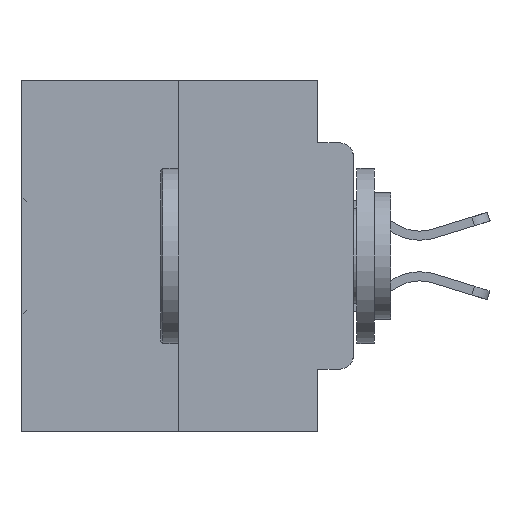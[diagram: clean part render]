
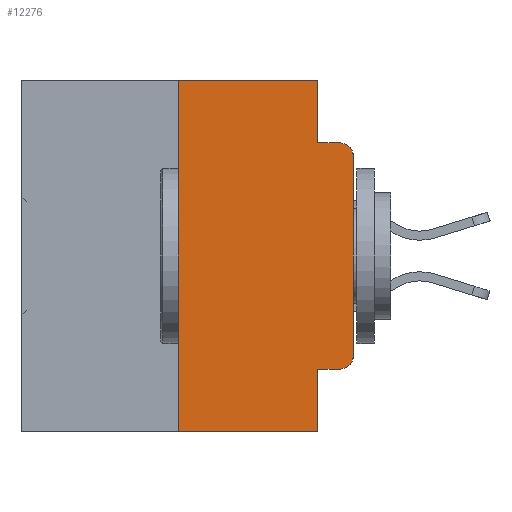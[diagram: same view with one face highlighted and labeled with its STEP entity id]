
A CAD part, left-side view. The second image highlights one B-rep face of the part: STEP entity #12276.
In plain terms, the highlighted planar face has unit normal (-1, 0, 0).
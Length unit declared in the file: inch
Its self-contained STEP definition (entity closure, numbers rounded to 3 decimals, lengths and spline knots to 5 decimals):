
#184 = CARTESIAN_POINT ( 'NONE',  ( 0., 0.02, -0.4115 ) ) ;
#1224 = AXIS2_PLACEMENT_3D ( 'NONE', #18841, #11108, #29218 ) ;
#1519 = ORIENTED_EDGE ( 'NONE', *, *, #25616, .T. ) ;
#1981 = ORIENTED_EDGE ( 'NONE', *, *, #29517, .F. ) ;
#2162 = DIRECTION ( 'NONE',  ( 0., -1., 0. ) ) ;
#2672 = CIRCLE ( 'NONE', #17789, 0.02 ) ;
#2979 = CARTESIAN_POINT ( 'NONE',  ( 0., 0.051, -0.0885 ) ) ;
#3383 = LINE ( 'NONE', #22987, #22512 ) ;
#3683 = VECTOR ( 'NONE', #31004, 39.37008 ) ;
#4195 = CARTESIAN_POINT ( 'NONE',  ( 0., 0., -0.1085 ) ) ;
#4209 = LINE ( 'NONE', #6127, #18863 ) ;
#4458 = CARTESIAN_POINT ( 'NONE',  ( 0., 0.02, -0.1085 ) ) ;
#4863 = VERTEX_POINT ( 'NONE', #7404 ) ;
#4993 = LINE ( 'NONE', #8942, #24950 ) ;
#5609 = DIRECTION ( 'NONE',  ( 0., -1., 0. ) ) ;
#5729 = VECTOR ( 'NONE', #16013, 39.37008 ) ;
#5787 = VERTEX_POINT ( 'NONE', #30250 ) ;
#5903 = VERTEX_POINT ( 'NONE', #7399 ) ;
#6127 = CARTESIAN_POINT ( 'NONE',  ( 0., 0.051, 0. ) ) ;
#6331 = CARTESIAN_POINT ( 'NONE',  ( 0., 0.02, -0.0885 ) ) ;
#6357 = DIRECTION ( 'NONE',  ( 0., 0., 1. ) ) ;
#6888 = LINE ( 'NONE', #2979, #33514 ) ;
#7072 = DIRECTION ( 'NONE',  ( 0., 0., -1. ) ) ;
#7381 = EDGE_CURVE ( 'NONE', #21571, #5903, #15150, .T. ) ;
#7399 = CARTESIAN_POINT ( 'NONE',  ( 0., 0.051, -0.5 ) ) ;
#7404 = CARTESIAN_POINT ( 'NONE',  ( 0., 0.051, -0.0885 ) ) ;
#7880 = FACE_OUTER_BOUND ( 'NONE', #33352, .T. ) ;
#8194 = VECTOR ( 'NONE', #9558, 39.37008 ) ;
#8215 = EDGE_CURVE ( 'NONE', #5787, #15349, #24443, .T. ) ;
#8376 = PLANE ( 'NONE',  #1224 ) ;
#8942 = CARTESIAN_POINT ( 'NONE',  ( 0., 0.25, 0. ) ) ;
#9016 = EDGE_CURVE ( 'NONE', #4863, #23266, #6888, .T. ) ;
#9089 = LINE ( 'NONE', #32446, #22137 ) ;
#9558 = DIRECTION ( 'NONE',  ( 0., -1., 0. ) ) ;
#11108 = DIRECTION ( 'NONE',  ( 1., 0., 0. ) ) ;
#11273 = EDGE_CURVE ( 'NONE', #15349, #16088, #2672, .T. ) ;
#12276 = ADVANCED_FACE ( 'NONE', ( #7880 ), #8376, .F. ) ;
#12431 = EDGE_CURVE ( 'NONE', #16143, #4863, #9089, .T. ) ;
#12445 = DIRECTION ( 'NONE',  ( -1., 0., 0. ) ) ;
#13007 = ORIENTED_EDGE ( 'NONE', *, *, #8215, .T. ) ;
#13732 = EDGE_CURVE ( 'NONE', #21571, #32492, #4993, .T. ) ;
#14284 = CARTESIAN_POINT ( 'NONE',  ( 0., 0.25, 0. ) ) ;
#14655 = ORIENTED_EDGE ( 'NONE', *, *, #11273, .T. ) ;
#15150 = LINE ( 'NONE', #32286, #8194 ) ;
#15349 = VERTEX_POINT ( 'NONE', #184 ) ;
#16013 = DIRECTION ( 'NONE',  ( 0., 0., 1. ) ) ;
#16088 = VERTEX_POINT ( 'NONE', #21189 ) ;
#16143 = VERTEX_POINT ( 'NONE', #24029 ) ;
#16516 = CIRCLE ( 'NONE', #30756, 0.02 ) ;
#17789 = AXIS2_PLACEMENT_3D ( 'NONE', #27961, #12445, #30515 ) ;
#18751 = LINE ( 'NONE', #30981, #5729 ) ;
#18841 = CARTESIAN_POINT ( 'NONE',  ( 0., 0.473, 0. ) ) ;
#18863 = VECTOR ( 'NONE', #24318, 39.37008 ) ;
#19879 = EDGE_CURVE ( 'NONE', #32492, #16143, #3383, .T. ) ;
#20706 = ORIENTED_EDGE ( 'NONE', *, *, #19879, .F. ) ;
#21189 = CARTESIAN_POINT ( 'NONE',  ( 0., 0., -0.3915 ) ) ;
#21571 = VERTEX_POINT ( 'NONE', #32174 ) ;
#22137 = VECTOR ( 'NONE', #29890, 39.37008 ) ;
#22343 = ORIENTED_EDGE ( 'NONE', *, *, #13732, .F. ) ;
#22512 = VECTOR ( 'NONE', #2162, 39.37008 ) ;
#22667 = DIRECTION ( 'NONE',  ( -1., 0., 0. ) ) ;
#22987 = CARTESIAN_POINT ( 'NONE',  ( 0., 0.473, 0. ) ) ;
#23266 = VERTEX_POINT ( 'NONE', #6331 ) ;
#24029 = CARTESIAN_POINT ( 'NONE',  ( 0., 0.051, 0. ) ) ;
#24318 = DIRECTION ( 'NONE',  ( 0., 0., -1. ) ) ;
#24443 = LINE ( 'NONE', #28452, #3683 ) ;
#24950 = VECTOR ( 'NONE', #6357, 39.37008 ) ;
#25616 = EDGE_CURVE ( 'NONE', #16088, #26536, #18751, .T. ) ;
#26536 = VERTEX_POINT ( 'NONE', #4195 ) ;
#27162 = ORIENTED_EDGE ( 'NONE', *, *, #9016, .F. ) ;
#27961 = CARTESIAN_POINT ( 'NONE',  ( 0., 0.02, -0.3915 ) ) ;
#28452 = CARTESIAN_POINT ( 'NONE',  ( 0., 0.051, -0.4115 ) ) ;
#28579 = EDGE_CURVE ( 'NONE', #26536, #23266, #16516, .T. ) ;
#28752 = ORIENTED_EDGE ( 'NONE', *, *, #12431, .F. ) ;
#29218 = DIRECTION ( 'NONE',  ( 0., 0., -1. ) ) ;
#29517 = EDGE_CURVE ( 'NONE', #5787, #5903, #4209, .T. ) ;
#29890 = DIRECTION ( 'NONE',  ( 0., 0., -1. ) ) ;
#29946 = ORIENTED_EDGE ( 'NONE', *, *, #28579, .T. ) ;
#30250 = CARTESIAN_POINT ( 'NONE',  ( 0., 0.051, -0.4115 ) ) ;
#30515 = DIRECTION ( 'NONE',  ( 0., 0., -1. ) ) ;
#30756 = AXIS2_PLACEMENT_3D ( 'NONE', #4458, #22667, #7072 ) ;
#30981 = CARTESIAN_POINT ( 'NONE',  ( 0., 0., 0. ) ) ;
#31004 = DIRECTION ( 'NONE',  ( 0., -1., 0. ) ) ;
#32174 = CARTESIAN_POINT ( 'NONE',  ( 0., 0.25, -0.5 ) ) ;
#32286 = CARTESIAN_POINT ( 'NONE',  ( 0., 0.473, -0.5 ) ) ;
#32446 = CARTESIAN_POINT ( 'NONE',  ( 0., 0.051, 0. ) ) ;
#32492 = VERTEX_POINT ( 'NONE', #14284 ) ;
#33145 = ORIENTED_EDGE ( 'NONE', *, *, #7381, .T. ) ;
#33352 = EDGE_LOOP ( 'NONE', ( #1519, #29946, #27162, #28752, #20706, #22343, #33145, #1981, #13007, #14655 ) ) ;
#33514 = VECTOR ( 'NONE', #5609, 39.37008 ) ;
